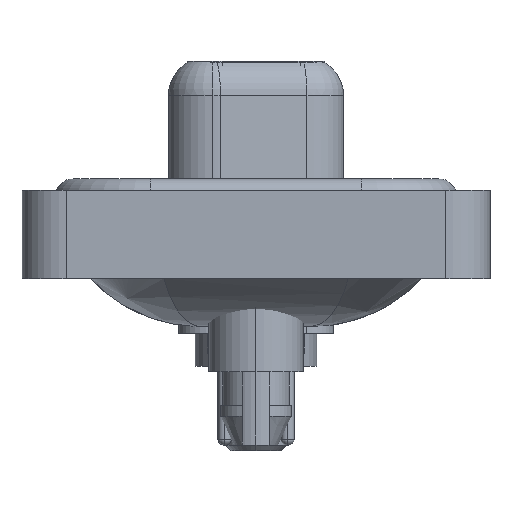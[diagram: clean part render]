
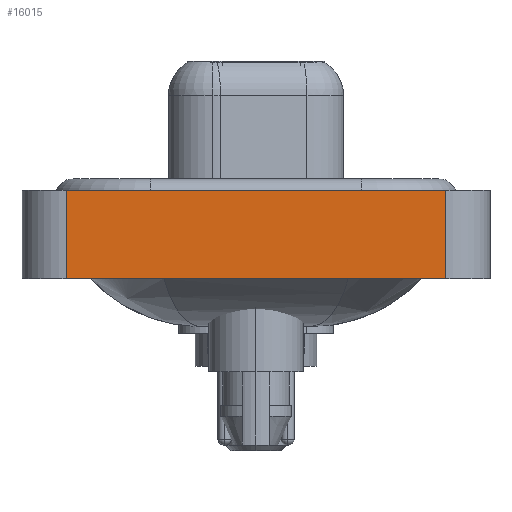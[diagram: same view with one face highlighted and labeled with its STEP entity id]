
A CAD part, left-side view. The second image highlights one B-rep face of the part: STEP entity #16015.
In plain terms, the highlighted planar face has unit normal (-1, 0, 0).
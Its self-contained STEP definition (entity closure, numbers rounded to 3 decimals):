
#546 = CARTESIAN_POINT ( 'NONE',  ( -7.3, 8.55, 0.4 ) ) ;
#820 = CARTESIAN_POINT ( 'NONE',  ( -7.3, 8.55, -3.6 ) ) ;
#926 = DIRECTION ( 'NONE',  ( 0., 0., 1. ) ) ;
#1890 = VERTEX_POINT ( 'NONE', #3831 ) ;
#2784 = VERTEX_POINT ( 'NONE', #20624 ) ;
#3391 = AXIS2_PLACEMENT_3D ( 'NONE', #19169, #15600, #20641 ) ;
#3639 = VECTOR ( 'NONE', #11117, 1000. ) ;
#3831 = CARTESIAN_POINT ( 'NONE',  ( -7.3, -8.55, 0.4 ) ) ;
#3868 = LINE ( 'NONE', #6991, #12078 ) ;
#6991 = CARTESIAN_POINT ( 'NONE',  ( -7.3, -8.55, -3.6 ) ) ;
#7038 = FACE_OUTER_BOUND ( 'NONE', #15908, .T. ) ;
#8058 = EDGE_CURVE ( 'NONE', #2784, #1890, #3868, .T. ) ;
#8280 = ORIENTED_EDGE ( 'NONE', *, *, #8058, .T. ) ;
#10520 = DIRECTION ( 'NONE',  ( 0., 0., 1. ) ) ;
#11117 = DIRECTION ( 'NONE',  ( 0., -1., 0. ) ) ;
#11402 = EDGE_CURVE ( 'NONE', #12525, #2784, #18560, .T. ) ;
#12048 = PLANE ( 'NONE',  #3391 ) ;
#12078 = VECTOR ( 'NONE', #10520, 1000. ) ;
#12525 = VERTEX_POINT ( 'NONE', #18619 ) ;
#12836 = EDGE_CURVE ( 'NONE', #16565, #1890, #19753, .T. ) ;
#14574 = DIRECTION ( 'NONE',  ( 0., -1., 0. ) ) ;
#14880 = CARTESIAN_POINT ( 'NONE',  ( -7.3, -8.55, -3.6 ) ) ;
#15600 = DIRECTION ( 'NONE',  ( -1., 0., 0. ) ) ;
#15908 = EDGE_LOOP ( 'NONE', ( #8280, #19204, #22431, #20387 ) ) ;
#16015 = ADVANCED_FACE ( 'NONE', ( #7038 ), #12048, .T. ) ;
#16565 = VERTEX_POINT ( 'NONE', #546 ) ;
#18538 = EDGE_CURVE ( 'NONE', #12525, #16565, #21652, .T. ) ;
#18560 = LINE ( 'NONE', #14880, #3639 ) ;
#18619 = CARTESIAN_POINT ( 'NONE',  ( -7.3, 8.55, -3.6 ) ) ;
#19169 = CARTESIAN_POINT ( 'NONE',  ( -7.3, -8.55, -3.6 ) ) ;
#19204 = ORIENTED_EDGE ( 'NONE', *, *, #12836, .F. ) ;
#19753 = LINE ( 'NONE', #21348, #21273 ) ;
#20315 = VECTOR ( 'NONE', #926, 1000. ) ;
#20387 = ORIENTED_EDGE ( 'NONE', *, *, #11402, .T. ) ;
#20624 = CARTESIAN_POINT ( 'NONE',  ( -7.3, -8.55, -3.6 ) ) ;
#20641 = DIRECTION ( 'NONE',  ( 0., 0., 1. ) ) ;
#21273 = VECTOR ( 'NONE', #14574, 1000. ) ;
#21348 = CARTESIAN_POINT ( 'NONE',  ( -7.3, -8.55, 0.4 ) ) ;
#21652 = LINE ( 'NONE', #820, #20315 ) ;
#22431 = ORIENTED_EDGE ( 'NONE', *, *, #18538, .F. ) ;
